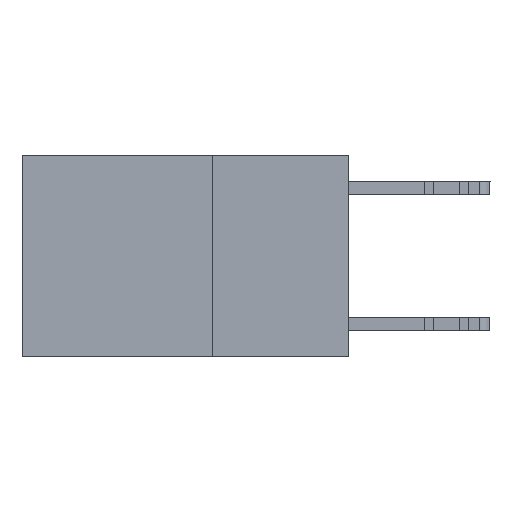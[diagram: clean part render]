
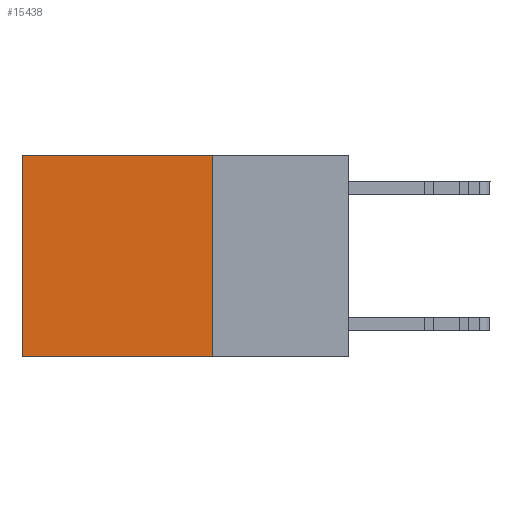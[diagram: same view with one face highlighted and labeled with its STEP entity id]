
A CAD part, left-side view. The second image highlights one B-rep face of the part: STEP entity #15438.
In plain terms, the highlighted planar face has unit normal (-1, 0, 0).
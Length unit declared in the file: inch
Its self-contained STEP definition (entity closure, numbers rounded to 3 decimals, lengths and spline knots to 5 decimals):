
#506 = ORIENTED_EDGE ( 'NONE', *, *, #18842, .T. ) ;
#608 = VERTEX_POINT ( 'NONE', #28360 ) ;
#1100 = VECTOR ( 'NONE', #15612, 39.37008 ) ;
#1431 = CARTESIAN_POINT ( 'NONE',  ( 0.2625, 0.25, 0. ) ) ;
#2571 = VECTOR ( 'NONE', #14646, 39.37008 ) ;
#4325 = ORIENTED_EDGE ( 'NONE', *, *, #25040, .F. ) ;
#4625 = EDGE_CURVE ( 'NONE', #26456, #608, #18601, .T. ) ;
#5171 = VECTOR ( 'NONE', #20183, 39.37008 ) ;
#6084 = CARTESIAN_POINT ( 'NONE',  ( 0.2625, 0.25, -0.37 ) ) ;
#6201 = EDGE_LOOP ( 'NONE', ( #30243, #4325, #8844, #506 ) ) ;
#7231 = EDGE_CURVE ( 'NONE', #19101, #12951, #18190, .T. ) ;
#8844 = ORIENTED_EDGE ( 'NONE', *, *, #7231, .F. ) ;
#10156 = CARTESIAN_POINT ( 'NONE',  ( 0.2625, 0.6, 0. ) ) ;
#10336 = LINE ( 'NONE', #21870, #2571 ) ;
#11029 = DIRECTION ( 'NONE',  ( 0., 0., -1. ) ) ;
#12503 = CARTESIAN_POINT ( 'NONE',  ( 0.2625, 0.25, -0.37 ) ) ;
#12951 = VERTEX_POINT ( 'NONE', #12503 ) ;
#13671 = VECTOR ( 'NONE', #25693, 39.37008 ) ;
#14468 = CARTESIAN_POINT ( 'NONE',  ( 0.2625, 0.25, 0. ) ) ;
#14646 = DIRECTION ( 'NONE',  ( 0., 1., 0. ) ) ;
#15438 = ADVANCED_FACE ( 'NONE', ( #20091 ), #29499, .F. ) ;
#15612 = DIRECTION ( 'NONE',  ( 0., 1., 0. ) ) ;
#16297 = CARTESIAN_POINT ( 'NONE',  ( 0.2625, 0.6, 0. ) ) ;
#18190 = LINE ( 'NONE', #1431, #5171 ) ;
#18601 = LINE ( 'NONE', #16297, #13671 ) ;
#18842 = EDGE_CURVE ( 'NONE', #19101, #26456, #10336, .T. ) ;
#19101 = VERTEX_POINT ( 'NONE', #14468 ) ;
#20091 = FACE_OUTER_BOUND ( 'NONE', #6201, .T. ) ;
#20183 = DIRECTION ( 'NONE',  ( 0., 0., -1. ) ) ;
#21870 = CARTESIAN_POINT ( 'NONE',  ( 0.2625, 0.25, 0. ) ) ;
#22876 = CARTESIAN_POINT ( 'NONE',  ( 0.2625, 0.25, 0. ) ) ;
#24502 = AXIS2_PLACEMENT_3D ( 'NONE', #22876, #27037, #11029 ) ;
#25040 = EDGE_CURVE ( 'NONE', #12951, #608, #27168, .T. ) ;
#25693 = DIRECTION ( 'NONE',  ( 0., 0., -1. ) ) ;
#26456 = VERTEX_POINT ( 'NONE', #10156 ) ;
#27037 = DIRECTION ( 'NONE',  ( 1., 0., 0. ) ) ;
#27168 = LINE ( 'NONE', #6084, #1100 ) ;
#28360 = CARTESIAN_POINT ( 'NONE',  ( 0.2625, 0.6, -0.37 ) ) ;
#29499 = PLANE ( 'NONE',  #24502 ) ;
#30243 = ORIENTED_EDGE ( 'NONE', *, *, #4625, .T. ) ;
